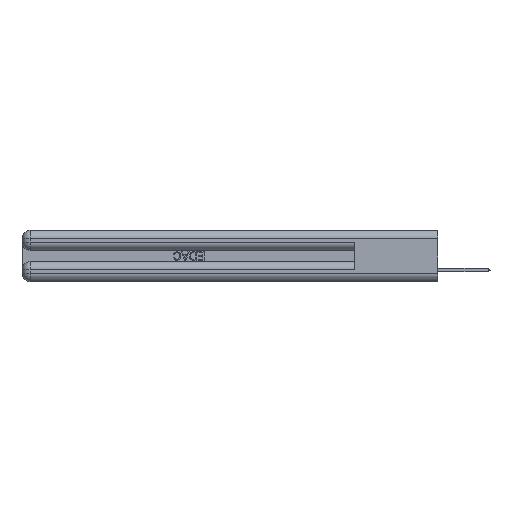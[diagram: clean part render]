
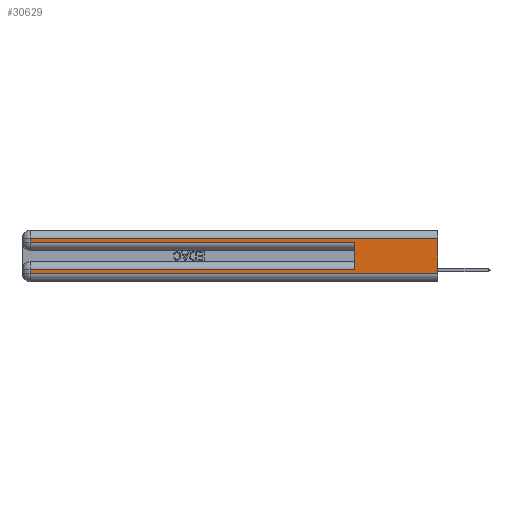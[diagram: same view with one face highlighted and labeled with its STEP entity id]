
A CAD part, left-side view. The second image highlights one B-rep face of the part: STEP entity #30629.
In plain terms, the highlighted planar face has unit normal (-1, 0, 0).
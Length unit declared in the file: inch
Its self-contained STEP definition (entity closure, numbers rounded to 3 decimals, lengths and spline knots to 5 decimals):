
#90 = EDGE_CURVE ( 'NONE', #8809, #43109, #32256, .T. ) ;
#1170 = FACE_OUTER_BOUND ( 'NONE', #33115, .T. ) ;
#4231 = EDGE_CURVE ( 'NONE', #41941, #41512, #24224, .T. ) ;
#4311 = CARTESIAN_POINT ( 'NONE',  ( 0., 0., 0.085 ) ) ;
#5482 = VECTOR ( 'NONE', #11887, 39.37008 ) ;
#5733 = LINE ( 'NONE', #14286, #43035 ) ;
#5827 = CARTESIAN_POINT ( 'NONE',  ( 0., 0.6, 0.285 ) ) ;
#6328 = ORIENTED_EDGE ( 'NONE', *, *, #11471, .T. ) ;
#7325 = VECTOR ( 'NONE', #13236, 39.37008 ) ;
#7389 = ORIENTED_EDGE ( 'NONE', *, *, #26284, .F. ) ;
#7555 = LINE ( 'NONE', #41054, #27410 ) ;
#7899 = LINE ( 'NONE', #23006, #24918 ) ;
#8809 = VERTEX_POINT ( 'NONE', #21421 ) ;
#10278 = CARTESIAN_POINT ( 'NONE',  ( 0., 0., 0.06 ) ) ;
#10839 = EDGE_CURVE ( 'NONE', #39290, #37860, #5733, .T. ) ;
#11471 = EDGE_CURVE ( 'NONE', #39290, #21585, #29870, .T. ) ;
#11887 = DIRECTION ( 'NONE',  ( 0., -1., 0. ) ) ;
#12074 = DIRECTION ( 'NONE',  ( 0., 0., -1. ) ) ;
#12729 = DIRECTION ( 'NONE',  ( 0., 0., -1. ) ) ;
#13236 = DIRECTION ( 'NONE',  ( 0., 1., 0. ) ) ;
#13672 = LINE ( 'NONE', #10278, #25099 ) ;
#14286 = CARTESIAN_POINT ( 'NONE',  ( 0., 0., 0.37 ) ) ;
#14865 = ORIENTED_EDGE ( 'NONE', *, *, #42074, .T. ) ;
#15683 = EDGE_CURVE ( 'NONE', #43109, #17739, #7555, .T. ) ;
#15743 = CARTESIAN_POINT ( 'NONE',  ( 0., 0., 0.285 ) ) ;
#16594 = DIRECTION ( 'NONE',  ( 0., 0., -1. ) ) ;
#17739 = VERTEX_POINT ( 'NONE', #22371 ) ;
#20164 = ORIENTED_EDGE ( 'NONE', *, *, #90, .T. ) ;
#21421 = CARTESIAN_POINT ( 'NONE',  ( 0., 0.6, 0.085 ) ) ;
#21585 = VERTEX_POINT ( 'NONE', #36408 ) ;
#22303 = VECTOR ( 'NONE', #39489, 39.37008 ) ;
#22371 = CARTESIAN_POINT ( 'NONE',  ( 0., 2.94, 0.06 ) ) ;
#23006 = CARTESIAN_POINT ( 'NONE',  ( 0., 0.6, 0.145 ) ) ;
#24224 = LINE ( 'NONE', #15743, #5482 ) ;
#24918 = VECTOR ( 'NONE', #40359, 39.37008 ) ;
#25099 = VECTOR ( 'NONE', #37722, 39.37008 ) ;
#25138 = VECTOR ( 'NONE', #12729, 39.37008 ) ;
#26284 = EDGE_CURVE ( 'NONE', #8809, #41512, #7899, .T. ) ;
#26589 = ORIENTED_EDGE ( 'NONE', *, *, #15683, .T. ) ;
#27410 = VECTOR ( 'NONE', #40017, 39.37008 ) ;
#27503 = PLANE ( 'NONE',  #33548 ) ;
#27812 = ORIENTED_EDGE ( 'NONE', *, *, #4231, .T. ) ;
#29870 = LINE ( 'NONE', #34877, #7325 ) ;
#30242 = CARTESIAN_POINT ( 'NONE',  ( 0., 2.94, 0.285 ) ) ;
#30267 = CARTESIAN_POINT ( 'NONE',  ( 0., 0., 0.37 ) ) ;
#30390 = CARTESIAN_POINT ( 'NONE',  ( 0., 2.94, 0.37 ) ) ;
#30583 = CARTESIAN_POINT ( 'NONE',  ( 0., 0., 0.06 ) ) ;
#30629 = ADVANCED_FACE ( 'NONE', ( #1170 ), #27503, .F. ) ;
#32256 = LINE ( 'NONE', #4311, #22303 ) ;
#33115 = EDGE_LOOP ( 'NONE', ( #43854, #6328, #36537, #27812, #7389, #20164, #26589, #14865 ) ) ;
#33548 = AXIS2_PLACEMENT_3D ( 'NONE', #30267, #37438, #16594 ) ;
#33815 = CARTESIAN_POINT ( 'NONE',  ( 0., 2.94, 0.085 ) ) ;
#34877 = CARTESIAN_POINT ( 'NONE',  ( 0., 0., 0.31 ) ) ;
#36408 = CARTESIAN_POINT ( 'NONE',  ( 0., 2.94, 0.31 ) ) ;
#36537 = ORIENTED_EDGE ( 'NONE', *, *, #40807, .T. ) ;
#37438 = DIRECTION ( 'NONE',  ( 1., 0., 0. ) ) ;
#37722 = DIRECTION ( 'NONE',  ( 0., -1., 0. ) ) ;
#37860 = VERTEX_POINT ( 'NONE', #30583 ) ;
#38894 = LINE ( 'NONE', #30390, #25138 ) ;
#39290 = VERTEX_POINT ( 'NONE', #42834 ) ;
#39489 = DIRECTION ( 'NONE',  ( 0., 1., 0. ) ) ;
#40017 = DIRECTION ( 'NONE',  ( 0., 0., -1. ) ) ;
#40359 = DIRECTION ( 'NONE',  ( 0., 0., 1. ) ) ;
#40807 = EDGE_CURVE ( 'NONE', #21585, #41941, #38894, .T. ) ;
#41054 = CARTESIAN_POINT ( 'NONE',  ( 0., 2.94, 0.37 ) ) ;
#41512 = VERTEX_POINT ( 'NONE', #5827 ) ;
#41941 = VERTEX_POINT ( 'NONE', #30242 ) ;
#42074 = EDGE_CURVE ( 'NONE', #17739, #37860, #13672, .T. ) ;
#42834 = CARTESIAN_POINT ( 'NONE',  ( 0., 0., 0.31 ) ) ;
#43035 = VECTOR ( 'NONE', #12074, 39.37008 ) ;
#43109 = VERTEX_POINT ( 'NONE', #33815 ) ;
#43854 = ORIENTED_EDGE ( 'NONE', *, *, #10839, .F. ) ;
